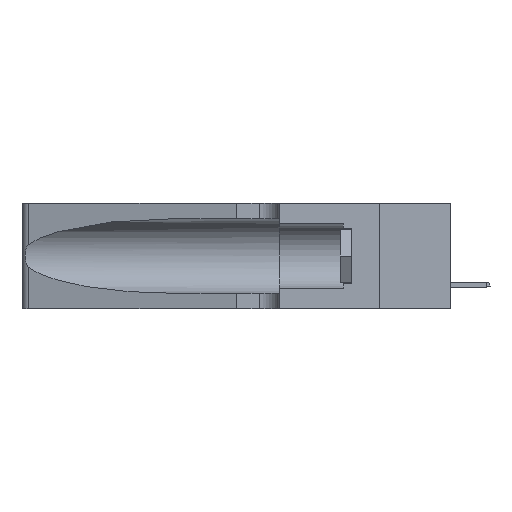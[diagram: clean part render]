
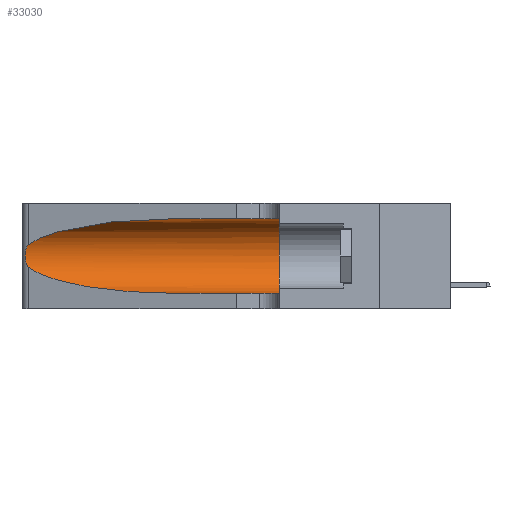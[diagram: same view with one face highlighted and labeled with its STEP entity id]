
A CAD part, left-side view. The second image highlights one B-rep face of the part: STEP entity #33030.
In plain terms, the highlighted cylindrical face has radius 3.308 mm (diameter 6.617 mm), a partial arc.
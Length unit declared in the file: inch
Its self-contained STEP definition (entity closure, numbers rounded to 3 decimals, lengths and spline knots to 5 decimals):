
#1220 = VERTEX_POINT ( 'NONE', #17681 ) ;
#1415 = VERTEX_POINT ( 'NONE', #7899 ) ;
#1670 = CARTESIAN_POINT ( 'NONE',  ( 0.25854, 1.2359, 0.20912 ) ) ;
#2248 = VERTEX_POINT ( 'NONE', #30028 ) ;
#3280 = CARTESIAN_POINT ( 'NONE',  ( 0.1305, 1.61858, 0.31525 ) ) ;
#4453 = FACE_OUTER_BOUND ( 'NONE', #29847, .T. ) ;
#4523 = ORIENTED_EDGE ( 'NONE', *, *, #13453, .T. ) ;
#4553 = CARTESIAN_POINT ( 'NONE',  ( 0.25555, 1.22994, 0.2215 ) ) ;
#5362 = CARTESIAN_POINT ( 'NONE',  ( 0.2373, 1.15595, 0.08982 ) ) ;
#6224 = CARTESIAN_POINT ( 'NONE',  ( 0.1305, 0.35, 0.185 ) ) ;
#6898 = CARTESIAN_POINT ( 'NONE',  ( 0.26075, 1.23896, 0.19203 ) ) ;
#7079 = CARTESIAN_POINT ( 'NONE',  ( 0.25555, 1.22993, 0.14849 ) ) ;
#7638 = ORIENTED_EDGE ( 'NONE', *, *, #11510, .T. ) ;
#7899 = CARTESIAN_POINT ( 'NONE',  ( 0.1305, 0.35, 0.31525 ) ) ;
#8872 = DIRECTION ( 'NONE',  ( 0., -1., 0. ) ) ;
#8971 =( BOUNDED_CURVE ( )  B_SPLINE_CURVE ( 3, ( #10648, #35419, #29494, #23875 ),
 .UNSPECIFIED., .F., .T. ) 
 B_SPLINE_CURVE_WITH_KNOTS ( ( 4, 4 ),
 ( 1.5708, 2.84003 ),
 .UNSPECIFIED. ) 
 CURVE ( )  GEOMETRIC_REPRESENTATION_ITEM ( )  RATIONAL_B_SPLINE_CURVE ( ( 1., 0.87, 0.87, 1. ) ) 
 REPRESENTATION_ITEM ( '' )  );
#9602 = CARTESIAN_POINT ( 'NONE',  ( 0.25487, 1.22718, 0.22369 ) ) ;
#10648 = CARTESIAN_POINT ( 'NONE',  ( 0.1305, 0.72297, 0.31525 ) ) ;
#10804 = CARTESIAN_POINT ( 'NONE',  ( 0.25487, 1.22718, 0.14631 ) ) ;
#11486 = EDGE_CURVE ( 'NONE', #1415, #2248, #22498, .T. ) ;
#11510 = EDGE_CURVE ( 'NONE', #1220, #2248, #33167, .T. ) ;
#12688 = CARTESIAN_POINT ( 'NONE',  ( 0.26075, 1.23896, 0.178 ) ) ;
#12765 = DIRECTION ( 'NONE',  ( 0., -1., 0. ) ) ;
#13453 = EDGE_CURVE ( 'NONE', #19339, #27991, #28844, .T. ) ;
#13495 = CARTESIAN_POINT ( 'NONE',  ( 0.1305, 0.72297, 0.05475 ) ) ;
#14002 = DIRECTION ( 'NONE',  ( 0., 0., 1. ) ) ;
#14644 = LINE ( 'NONE', #3280, #17838 ) ;
#14798 = AXIS2_PLACEMENT_3D ( 'NONE', #35167, #12765, #29408 ) ;
#15577 = CARTESIAN_POINT ( 'NONE',  ( 0.25856, 1.23593, 0.16098 ) ) ;
#17681 = CARTESIAN_POINT ( 'NONE',  ( 0.1305, 0.72297, 0.05475 ) ) ;
#17746 =( BOUNDED_CURVE ( )  B_SPLINE_CURVE ( 3, ( #35540, #5362, #29442, #13495 ),
 .UNSPECIFIED., .F., .T. ) 
 B_SPLINE_CURVE_WITH_KNOTS ( ( 4, 4 ),
 ( 3.44316, 4.71239 ),
 .UNSPECIFIED. ) 
 CURVE ( )  GEOMETRIC_REPRESENTATION_ITEM ( )  RATIONAL_B_SPLINE_CURVE ( ( 1., 0.87, 0.87, 1. ) ) 
 REPRESENTATION_ITEM ( '' )  );
#17838 = VECTOR ( 'NONE', #8872, 39.37008 ) ;
#18111 = CARTESIAN_POINT ( 'NONE',  ( 0.25487, 1.22718, 0.14631 ) ) ;
#18712 = EDGE_CURVE ( 'NONE', #23328, #19339, #8971, .T. ) ;
#19339 = VERTEX_POINT ( 'NONE', #27962 ) ;
#20110 = ORIENTED_EDGE ( 'NONE', *, *, #11486, .F. ) ;
#20665 = CARTESIAN_POINT ( 'NONE',  ( 0.25639, 1.23184, 0.21858 ) ) ;
#21345 = AXIS2_PLACEMENT_3D ( 'NONE', #6224, #30469, #14002 ) ;
#21423 = EDGE_CURVE ( 'NONE', #23328, #1415, #14644, .T. ) ;
#22118 = EDGE_CURVE ( 'NONE', #27991, #1220, #17746, .T. ) ;
#22498 = CIRCLE ( 'NONE', #21345, 0.13025 ) ;
#22517 = DIRECTION ( 'NONE',  ( 0., -1., 0. ) ) ;
#22971 = ORIENTED_EDGE ( 'NONE', *, *, #22118, .T. ) ;
#23328 = VERTEX_POINT ( 'NONE', #26188 ) ;
#23546 = ORIENTED_EDGE ( 'NONE', *, *, #18712, .T. ) ;
#23875 = CARTESIAN_POINT ( 'NONE',  ( 0.25487, 1.22718, 0.22369 ) ) ;
#23896 = CARTESIAN_POINT ( 'NONE',  ( 0.25787, 1.23484, 0.2124 ) ) ;
#24154 = CYLINDRICAL_SURFACE ( 'NONE', #14798, 0.13025 ) ;
#24219 = VECTOR ( 'NONE', #22517, 39.37008 ) ;
#26188 = CARTESIAN_POINT ( 'NONE',  ( 0.1305, 0.72297, 0.31525 ) ) ;
#26247 = CARTESIAN_POINT ( 'NONE',  ( 0.25789, 1.23486, 0.15765 ) ) ;
#27962 = CARTESIAN_POINT ( 'NONE',  ( 0.25487, 1.22718, 0.22369 ) ) ;
#27991 = VERTEX_POINT ( 'NONE', #10804 ) ;
#28844 = B_SPLINE_CURVE_WITH_KNOTS ( 'NONE', 3,
 ( #9602, #4553, #20665, #23896, #1670, #31663, #6898, #12688, #28966, #15577, #26247, #34902, #7079, #18111 ),
 .UNSPECIFIED., .F., .F.,
 ( 4, 2, 2, 2, 2, 2, 4 ),
 ( 0., 0.00027, 0.00053, 0.00107, 0.0016, 0.00187, 0.00214 ),
 .UNSPECIFIED. ) ;
#28966 = CARTESIAN_POINT ( 'NONE',  ( 0.26017, 1.23833, 0.17102 ) ) ;
#29408 = DIRECTION ( 'NONE',  ( 0., 0., -1. ) ) ;
#29442 = CARTESIAN_POINT ( 'NONE',  ( 0.18966, 0.96281, 0.05475 ) ) ;
#29494 = CARTESIAN_POINT ( 'NONE',  ( 0.2373, 1.15595, 0.28018 ) ) ;
#29847 = EDGE_LOOP ( 'NONE', ( #23546, #4523, #22971, #7638, #20110, #34464 ) ) ;
#30028 = CARTESIAN_POINT ( 'NONE',  ( 0.1305, 0.35, 0.05475 ) ) ;
#30469 = DIRECTION ( 'NONE',  ( 0., 1., 0. ) ) ;
#30823 = CARTESIAN_POINT ( 'NONE',  ( 0.1305, 1.61858, 0.05475 ) ) ;
#31663 = CARTESIAN_POINT ( 'NONE',  ( 0.26018, 1.23835, 0.19895 ) ) ;
#33030 = ADVANCED_FACE ( 'NONE', ( #4453 ), #24154, .F. ) ;
#33167 = LINE ( 'NONE', #30823, #24219 ) ;
#34464 = ORIENTED_EDGE ( 'NONE', *, *, #21423, .F. ) ;
#34902 = CARTESIAN_POINT ( 'NONE',  ( 0.25639, 1.23186, 0.15144 ) ) ;
#35167 = CARTESIAN_POINT ( 'NONE',  ( 0.1305, 1.61858, 0.185 ) ) ;
#35419 = CARTESIAN_POINT ( 'NONE',  ( 0.18966, 0.96281, 0.31525 ) ) ;
#35540 = CARTESIAN_POINT ( 'NONE',  ( 0.25487, 1.22718, 0.14631 ) ) ;
